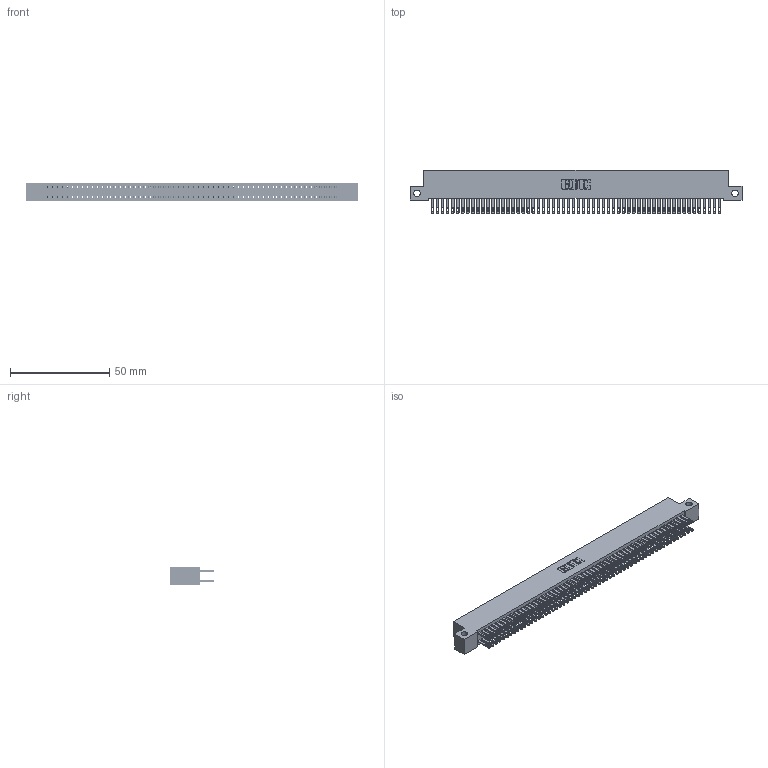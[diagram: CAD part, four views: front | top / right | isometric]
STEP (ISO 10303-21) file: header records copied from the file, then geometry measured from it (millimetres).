
FILE_DESCRIPTION (( 'STEP AP203' ), '1' );
FILE_NAME ('342-116-500-212.STEP', '2018-08-14T13:22:51', ( '' ), ( '' ), 'SwSTEP 2.0', 'SolidWorks 2016', '' );
FILE_SCHEMA (( 'CONFIG_CONTROL_DESIGN' ));
Length unit declared in the file: inch
Products named in the file (3): 342-116-500-212; 345-292-001_345-293-100; 342 Part_Side Mount
Assembly tree (117 placements, depth 2):
  342-116-500-212
    342 Part_Side Mount
    345-292-001_345-293-100  x116
Bounding box: 167.64 x 21.85 x 9.4 mm (x, y, z)
Volume: 15418.7 mm3; surface area: 26442.9 mm2
Topology: 117 solids, 117 shells, 5678 faces, 17351 edges, 11566 vertices
Faces by surface type: plane 3546, cylinder 2132
Entity records: 35045 total; most frequent: CARTESIAN_POINT 5786, ORIENTED_EDGE 5722, DIRECTION 4917, EDGE_CURVE 2861, VECTOR 2729, LINE 2729, VERTEX_POINT 1906, AXIS2_PLACEMENT_3D 1094
